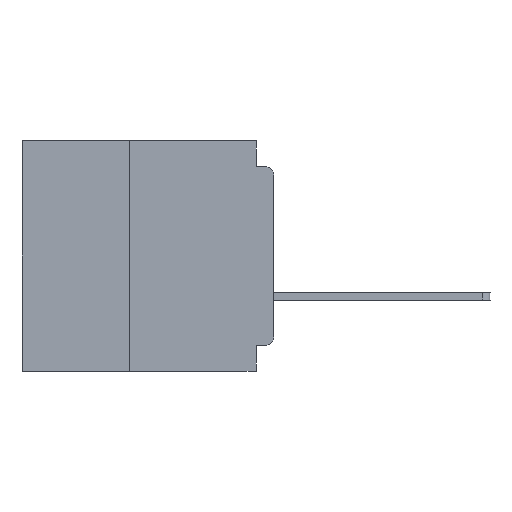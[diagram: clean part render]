
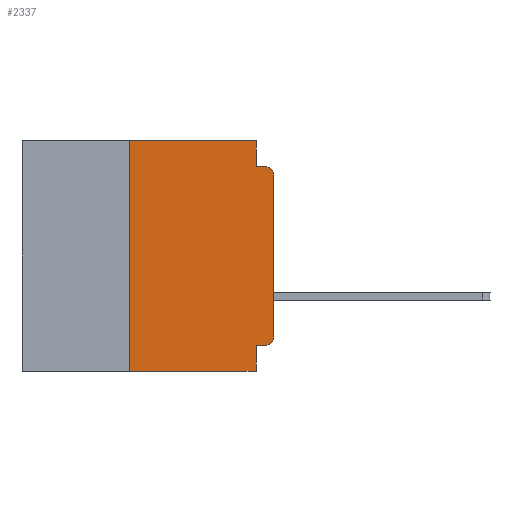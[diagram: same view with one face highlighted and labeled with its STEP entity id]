
A CAD part, left-side view. The second image highlights one B-rep face of the part: STEP entity #2337.
In plain terms, the highlighted planar face has unit normal (-1, 0, 0).
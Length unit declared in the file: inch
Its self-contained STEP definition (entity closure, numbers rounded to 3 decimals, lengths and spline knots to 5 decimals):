
#1506 = VERTEX_POINT ( 'NONE', #6696 ) ;
#1524 = DIRECTION ( 'NONE',  ( 0., -1., 0. ) ) ;
#1742 = CARTESIAN_POINT ( 'NONE',  ( 0., 0., -0.355 ) ) ;
#2337 = ADVANCED_FACE ( 'NONE', ( #48176 ), #36763, .F. ) ;
#3115 = CARTESIAN_POINT ( 'NONE',  ( 0., 0., -0.34 ) ) ;
#3426 = DIRECTION ( 'NONE',  ( 0., 0., -1. ) ) ;
#3993 = EDGE_CURVE ( 'NONE', #38131, #15312, #50659, .T. ) ;
#5132 = EDGE_CURVE ( 'NONE', #1506, #47317, #35506, .T. ) ;
#5148 = ORIENTED_EDGE ( 'NONE', *, *, #21813, .T. ) ;
#5893 = DIRECTION ( 'NONE',  ( -1., 0., 0. ) ) ;
#6241 = CARTESIAN_POINT ( 'NONE',  ( 0., 0.031, 0. ) ) ;
#6366 = ORIENTED_EDGE ( 'NONE', *, *, #27368, .F. ) ;
#6477 = CARTESIAN_POINT ( 'NONE',  ( 0., 0.031, -0.355 ) ) ;
#6696 = CARTESIAN_POINT ( 'NONE',  ( 0., 0.25, -0.4 ) ) ;
#6739 = LINE ( 'NONE', #41550, #18489 ) ;
#7610 = EDGE_CURVE ( 'NONE', #33924, #18936, #19801, .T. ) ;
#7633 = CARTESIAN_POINT ( 'NONE',  ( 0., 0.031, 0. ) ) ;
#8944 = ORIENTED_EDGE ( 'NONE', *, *, #7610, .F. ) ;
#12126 = VECTOR ( 'NONE', #39225, 39.37008 ) ;
#12986 = ORIENTED_EDGE ( 'NONE', *, *, #53846, .F. ) ;
#14613 = ORIENTED_EDGE ( 'NONE', *, *, #30307, .F. ) ;
#15312 = VERTEX_POINT ( 'NONE', #18613 ) ;
#15335 = DIRECTION ( 'NONE',  ( 0., 0., -1. ) ) ;
#16224 = VECTOR ( 'NONE', #18089, 39.37008 ) ;
#16320 = AXIS2_PLACEMENT_3D ( 'NONE', #43387, #17212, #47826 ) ;
#17212 = DIRECTION ( 'NONE',  ( -1., 0., 0. ) ) ;
#18089 = DIRECTION ( 'NONE',  ( 0., 0., 1. ) ) ;
#18489 = VECTOR ( 'NONE', #15335, 39.37008 ) ;
#18613 = CARTESIAN_POINT ( 'NONE',  ( 0., 0., -0.06 ) ) ;
#18936 = VERTEX_POINT ( 'NONE', #6241 ) ;
#19724 = VERTEX_POINT ( 'NONE', #55726 ) ;
#19801 = LINE ( 'NONE', #40844, #51927 ) ;
#20183 = LINE ( 'NONE', #7633, #52301 ) ;
#21018 = CIRCLE ( 'NONE', #16320, 0.015 ) ;
#21629 = CARTESIAN_POINT ( 'NONE',  ( 0., 0.031, -0.4 ) ) ;
#21813 = EDGE_CURVE ( 'NONE', #15312, #42278, #21018, .T. ) ;
#21922 = ORIENTED_EDGE ( 'NONE', *, *, #31745, .F. ) ;
#22568 = AXIS2_PLACEMENT_3D ( 'NONE', #32234, #5893, #36607 ) ;
#23625 = VECTOR ( 'NONE', #23860, 39.37008 ) ;
#23860 = DIRECTION ( 'NONE',  ( 0., 1., 0. ) ) ;
#27368 = EDGE_CURVE ( 'NONE', #44125, #29824, #35277, .T. ) ;
#29824 = VERTEX_POINT ( 'NONE', #6477 ) ;
#30307 = EDGE_CURVE ( 'NONE', #29824, #47317, #6739, .T. ) ;
#31163 = DIRECTION ( 'NONE',  ( 0., -1., 0. ) ) ;
#31707 = ORIENTED_EDGE ( 'NONE', *, *, #3993, .T. ) ;
#31745 = EDGE_CURVE ( 'NONE', #18936, #19724, #20183, .T. ) ;
#32234 = CARTESIAN_POINT ( 'NONE',  ( 0., 0.015, -0.34 ) ) ;
#33924 = VERTEX_POINT ( 'NONE', #43564 ) ;
#34789 = DIRECTION ( 'NONE',  ( 1., 0., 0. ) ) ;
#34916 = CARTESIAN_POINT ( 'NONE',  ( 0., 0.437, 0. ) ) ;
#35269 = CARTESIAN_POINT ( 'NONE',  ( 0., 0.015, -0.355 ) ) ;
#35277 = LINE ( 'NONE', #1742, #23625 ) ;
#35506 = LINE ( 'NONE', #37736, #12126 ) ;
#36607 = DIRECTION ( 'NONE',  ( 0., 0., -1. ) ) ;
#36763 = PLANE ( 'NONE',  #41587 ) ;
#37736 = CARTESIAN_POINT ( 'NONE',  ( 0., 0.437, -0.4 ) ) ;
#37778 = DIRECTION ( 'NONE',  ( 0., 0., -1. ) ) ;
#38131 = VERTEX_POINT ( 'NONE', #3115 ) ;
#39026 = VECTOR ( 'NONE', #54027, 39.37008 ) ;
#39225 = DIRECTION ( 'NONE',  ( 0., -1., 0. ) ) ;
#39820 = EDGE_CURVE ( 'NONE', #44125, #38131, #53804, .T. ) ;
#40844 = CARTESIAN_POINT ( 'NONE',  ( 0., 0.437, 0. ) ) ;
#41550 = CARTESIAN_POINT ( 'NONE',  ( 0., 0.031, -0.4 ) ) ;
#41587 = AXIS2_PLACEMENT_3D ( 'NONE', #34916, #34789, #37778 ) ;
#41701 = ORIENTED_EDGE ( 'NONE', *, *, #52693, .F. ) ;
#42278 = VERTEX_POINT ( 'NONE', #55224 ) ;
#43387 = CARTESIAN_POINT ( 'NONE',  ( 0., 0.015, -0.06 ) ) ;
#43564 = CARTESIAN_POINT ( 'NONE',  ( 0., 0.25, 0. ) ) ;
#44125 = VERTEX_POINT ( 'NONE', #35269 ) ;
#46227 = LINE ( 'NONE', #52889, #56388 ) ;
#47317 = VERTEX_POINT ( 'NONE', #21629 ) ;
#47826 = DIRECTION ( 'NONE',  ( 0., 0., -1. ) ) ;
#48176 = FACE_OUTER_BOUND ( 'NONE', #54682, .T. ) ;
#50659 = LINE ( 'NONE', #54158, #39026 ) ;
#51927 = VECTOR ( 'NONE', #1524, 39.37008 ) ;
#51967 = ORIENTED_EDGE ( 'NONE', *, *, #39820, .T. ) ;
#52301 = VECTOR ( 'NONE', #3426, 39.37008 ) ;
#52693 = EDGE_CURVE ( 'NONE', #1506, #33924, #53847, .T. ) ;
#52889 = CARTESIAN_POINT ( 'NONE',  ( 0., 0., -0.045 ) ) ;
#53207 = CARTESIAN_POINT ( 'NONE',  ( 0., 0.25, -0.4 ) ) ;
#53804 = CIRCLE ( 'NONE', #22568, 0.015 ) ;
#53846 = EDGE_CURVE ( 'NONE', #19724, #42278, #46227, .T. ) ;
#53847 = LINE ( 'NONE', #53207, #16224 ) ;
#54027 = DIRECTION ( 'NONE',  ( 0., 0., 1. ) ) ;
#54158 = CARTESIAN_POINT ( 'NONE',  ( 0., 0., 0. ) ) ;
#54682 = EDGE_LOOP ( 'NONE', ( #31707, #5148, #12986, #21922, #8944, #41701, #56393, #14613, #6366, #51967 ) ) ;
#55224 = CARTESIAN_POINT ( 'NONE',  ( 0., 0.015, -0.045 ) ) ;
#55726 = CARTESIAN_POINT ( 'NONE',  ( 0., 0.031, -0.045 ) ) ;
#56388 = VECTOR ( 'NONE', #31163, 39.37008 ) ;
#56393 = ORIENTED_EDGE ( 'NONE', *, *, #5132, .T. ) ;
